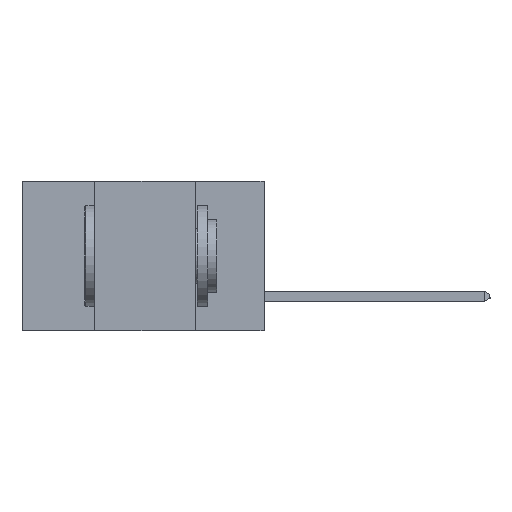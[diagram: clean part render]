
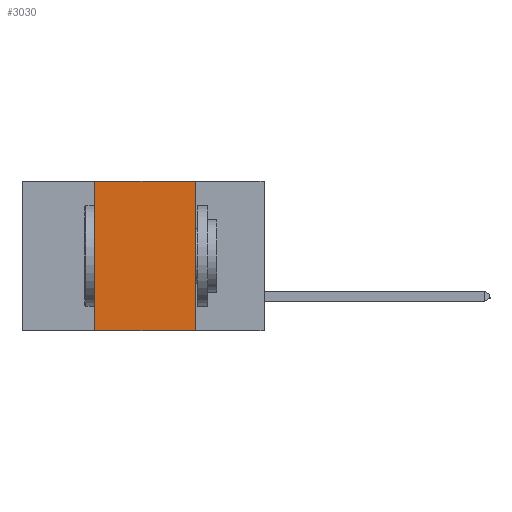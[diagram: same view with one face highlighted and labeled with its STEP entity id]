
A CAD part, left-side view. The second image highlights one B-rep face of the part: STEP entity #3030.
In plain terms, the highlighted planar face has unit normal (-1, 0, 0).
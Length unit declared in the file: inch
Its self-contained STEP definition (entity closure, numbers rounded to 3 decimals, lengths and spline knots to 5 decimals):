
#161 = DIRECTION ( 'NONE',  ( 0., -1., 0. ) ) ;
#452 = ORIENTED_EDGE ( 'NONE', *, *, #456, .F. ) ;
#456 = EDGE_CURVE ( 'NONE', #1987, #11193, #6921, .T. ) ;
#712 = EDGE_LOOP ( 'NONE', ( #452, #1269, #2093, #3233 ) ) ;
#992 = CARTESIAN_POINT ( 'NONE',  ( 0., 0.42, 0. ) ) ;
#1075 = DIRECTION ( 'NONE',  ( 0., -1., 0. ) ) ;
#1269 = ORIENTED_EDGE ( 'NONE', *, *, #5196, .F. ) ;
#1847 = AXIS2_PLACEMENT_3D ( 'NONE', #3515, #4625, #4678 ) ;
#1987 = VERTEX_POINT ( 'NONE', #3839 ) ;
#2035 = VECTOR ( 'NONE', #9354, 39.37008 ) ;
#2093 = ORIENTED_EDGE ( 'NONE', *, *, #11031, .F. ) ;
#2222 = VERTEX_POINT ( 'NONE', #4027 ) ;
#2269 = PLANE ( 'NONE',  #1847 ) ;
#3030 = ADVANCED_FACE ( 'NONE', ( #6485 ), #2269, .F. ) ;
#3233 = ORIENTED_EDGE ( 'NONE', *, *, #9257, .T. ) ;
#3350 = VECTOR ( 'NONE', #6572, 39.37008 ) ;
#3515 = CARTESIAN_POINT ( 'NONE',  ( 0., 0.6, 0. ) ) ;
#3656 = VECTOR ( 'NONE', #161, 39.37008 ) ;
#3839 = CARTESIAN_POINT ( 'NONE',  ( 0., 0.17, 0. ) ) ;
#4002 = VECTOR ( 'NONE', #1075, 39.37008 ) ;
#4027 = CARTESIAN_POINT ( 'NONE',  ( 0., 0.42, -0.37 ) ) ;
#4625 = DIRECTION ( 'NONE',  ( 1., 0., 0. ) ) ;
#4678 = DIRECTION ( 'NONE',  ( 0., 0., -1. ) ) ;
#5196 = EDGE_CURVE ( 'NONE', #6224, #1987, #6134, .T. ) ;
#5773 = CARTESIAN_POINT ( 'NONE',  ( 0., 0.6, -0.37 ) ) ;
#5839 = LINE ( 'NONE', #10953, #3350 ) ;
#6134 = LINE ( 'NONE', #8423, #3656 ) ;
#6224 = VERTEX_POINT ( 'NONE', #992 ) ;
#6441 = LINE ( 'NONE', #5773, #4002 ) ;
#6485 = FACE_OUTER_BOUND ( 'NONE', #712, .T. ) ;
#6572 = DIRECTION ( 'NONE',  ( 0., 0., 1. ) ) ;
#6921 = LINE ( 'NONE', #8620, #2035 ) ;
#8423 = CARTESIAN_POINT ( 'NONE',  ( 0., 0.6, 0. ) ) ;
#8620 = CARTESIAN_POINT ( 'NONE',  ( 0., 0.17, 0. ) ) ;
#9257 = EDGE_CURVE ( 'NONE', #2222, #11193, #6441, .T. ) ;
#9354 = DIRECTION ( 'NONE',  ( 0., 0., -1. ) ) ;
#10278 = CARTESIAN_POINT ( 'NONE',  ( 0., 0.17, -0.37 ) ) ;
#10953 = CARTESIAN_POINT ( 'NONE',  ( 0., 0.42, 0. ) ) ;
#11031 = EDGE_CURVE ( 'NONE', #2222, #6224, #5839, .T. ) ;
#11193 = VERTEX_POINT ( 'NONE', #10278 ) ;
